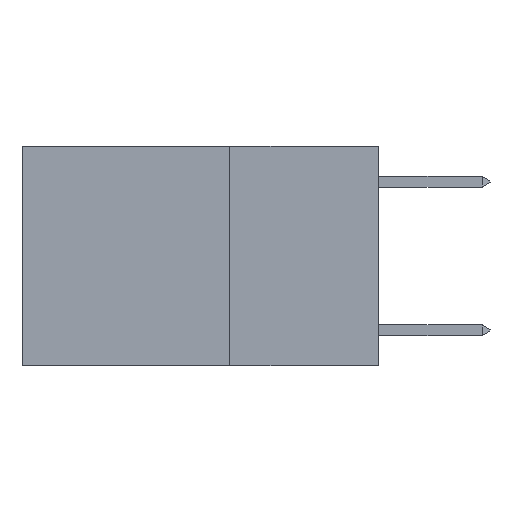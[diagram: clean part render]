
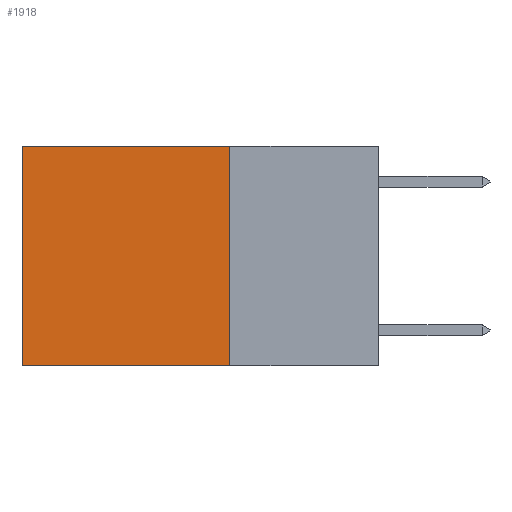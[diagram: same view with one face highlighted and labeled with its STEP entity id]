
A CAD part, left-side view. The second image highlights one B-rep face of the part: STEP entity #1918.
In plain terms, the highlighted planar face has unit normal (-1, 0, 0).
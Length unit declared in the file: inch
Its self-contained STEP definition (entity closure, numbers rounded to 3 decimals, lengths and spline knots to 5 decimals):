
#506 = EDGE_CURVE ( 'NONE', #26994, #22632, #16805, .T. ) ;
#1918 = ADVANCED_FACE ( 'NONE', ( #21046 ), #28749, .F. ) ;
#3502 = VERTEX_POINT ( 'NONE', #30501 ) ;
#4206 = CARTESIAN_POINT ( 'NONE',  ( 0.2625, 0.6, 0. ) ) ;
#5102 = DIRECTION ( 'NONE',  ( 0., 1., 0. ) ) ;
#7293 = DIRECTION ( 'NONE',  ( 0., 1., 0. ) ) ;
#8038 = VECTOR ( 'NONE', #5102, 39.37008 ) ;
#10717 = EDGE_CURVE ( 'NONE', #3502, #22632, #22549, .T. ) ;
#11139 = CARTESIAN_POINT ( 'NONE',  ( 0.2625, 0.25, 0. ) ) ;
#11953 = ORIENTED_EDGE ( 'NONE', *, *, #24290, .F. ) ;
#12374 = CARTESIAN_POINT ( 'NONE',  ( 0.2625, 0.25, -0.37 ) ) ;
#13522 = ORIENTED_EDGE ( 'NONE', *, *, #506, .T. ) ;
#13622 = EDGE_LOOP ( 'NONE', ( #13522, #14705, #11953, #24848 ) ) ;
#13868 = CARTESIAN_POINT ( 'NONE',  ( 0.2625, 0.25, 0. ) ) ;
#13874 = DIRECTION ( 'NONE',  ( 0., 0., -1. ) ) ;
#14705 = ORIENTED_EDGE ( 'NONE', *, *, #10717, .F. ) ;
#16805 = LINE ( 'NONE', #4206, #28745 ) ;
#19812 = CARTESIAN_POINT ( 'NONE',  ( 0.2625, 0.6, 0. ) ) ;
#21046 = FACE_OUTER_BOUND ( 'NONE', #13622, .T. ) ;
#21384 = DIRECTION ( 'NONE',  ( 0., 0., -1. ) ) ;
#21537 = CARTESIAN_POINT ( 'NONE',  ( 0.2625, 0.25, 0. ) ) ;
#22478 = LINE ( 'NONE', #24935, #8038 ) ;
#22517 = VECTOR ( 'NONE', #28132, 39.37008 ) ;
#22549 = LINE ( 'NONE', #12374, #25816 ) ;
#22632 = VERTEX_POINT ( 'NONE', #27808 ) ;
#23849 = VERTEX_POINT ( 'NONE', #11139 ) ;
#23885 = LINE ( 'NONE', #13868, #22517 ) ;
#24290 = EDGE_CURVE ( 'NONE', #23849, #3502, #23885, .T. ) ;
#24466 = AXIS2_PLACEMENT_3D ( 'NONE', #21537, #28422, #21384 ) ;
#24848 = ORIENTED_EDGE ( 'NONE', *, *, #25088, .T. ) ;
#24935 = CARTESIAN_POINT ( 'NONE',  ( 0.2625, 0.25, 0. ) ) ;
#25088 = EDGE_CURVE ( 'NONE', #23849, #26994, #22478, .T. ) ;
#25816 = VECTOR ( 'NONE', #7293, 39.37008 ) ;
#26994 = VERTEX_POINT ( 'NONE', #19812 ) ;
#27808 = CARTESIAN_POINT ( 'NONE',  ( 0.2625, 0.6, -0.37 ) ) ;
#28132 = DIRECTION ( 'NONE',  ( 0., 0., -1. ) ) ;
#28422 = DIRECTION ( 'NONE',  ( 1., 0., 0. ) ) ;
#28745 = VECTOR ( 'NONE', #13874, 39.37008 ) ;
#28749 = PLANE ( 'NONE',  #24466 ) ;
#30501 = CARTESIAN_POINT ( 'NONE',  ( 0.2625, 0.25, -0.37 ) ) ;
